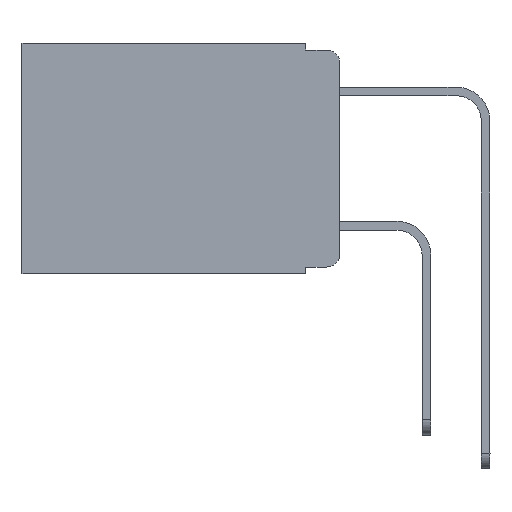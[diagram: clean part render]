
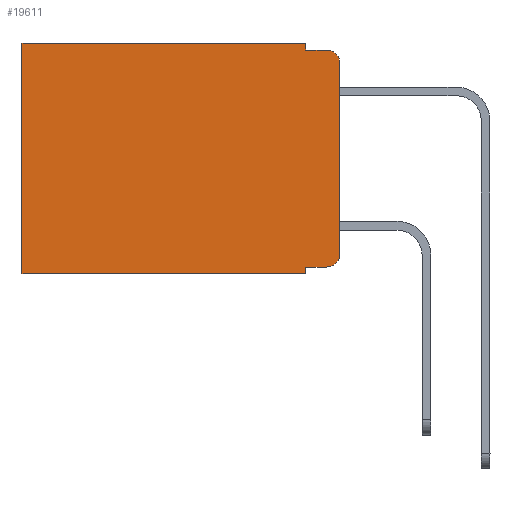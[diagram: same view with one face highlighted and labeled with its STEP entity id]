
A CAD part, left-side view. The second image highlights one B-rep face of the part: STEP entity #19611.
In plain terms, the highlighted planar face has unit normal (-1, 0, 0).
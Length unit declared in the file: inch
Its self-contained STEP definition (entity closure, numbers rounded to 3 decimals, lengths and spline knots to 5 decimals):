
#153 = VERTEX_POINT ( 'NONE', #23962 ) ;
#367 = ORIENTED_EDGE ( 'NONE', *, *, #16623, .T. ) ;
#507 = PLANE ( 'NONE',  #22811 ) ;
#697 = LINE ( 'NONE', #23389, #5428 ) ;
#757 = CARTESIAN_POINT ( 'NONE',  ( 0.298, 0., 0. ) ) ;
#948 = CIRCLE ( 'NONE', #19340, 0.02 ) ;
#1432 = CARTESIAN_POINT ( 'NONE',  ( 0.298, 0.051, -0.01 ) ) ;
#2094 = ORIENTED_EDGE ( 'NONE', *, *, #20021, .F. ) ;
#2096 = ORIENTED_EDGE ( 'NONE', *, *, #12876, .F. ) ;
#2594 = VECTOR ( 'NONE', #13783, 39.37008 ) ;
#2634 = DIRECTION ( 'NONE',  ( 0., 0., -1. ) ) ;
#2994 = DIRECTION ( 'NONE',  ( 0., 1., 0. ) ) ;
#3037 = ORIENTED_EDGE ( 'NONE', *, *, #12932, .F. ) ;
#3813 = CARTESIAN_POINT ( 'NONE',  ( 0.298, 0., -0.313 ) ) ;
#3879 = CARTESIAN_POINT ( 'NONE',  ( 0.298, 0.473, 0. ) ) ;
#4862 = ORIENTED_EDGE ( 'NONE', *, *, #23578, .T. ) ;
#5006 = DIRECTION ( 'NONE',  ( 0., 0., -1. ) ) ;
#5026 = VERTEX_POINT ( 'NONE', #20589 ) ;
#5389 = ORIENTED_EDGE ( 'NONE', *, *, #7988, .F. ) ;
#5428 = VECTOR ( 'NONE', #6217, 39.37008 ) ;
#6217 = DIRECTION ( 'NONE',  ( 0., 0., -1. ) ) ;
#7221 = VECTOR ( 'NONE', #14536, 39.37008 ) ;
#7294 = ORIENTED_EDGE ( 'NONE', *, *, #7670, .T. ) ;
#7316 = LINE ( 'NONE', #9185, #12214 ) ;
#7670 = EDGE_CURVE ( 'NONE', #18121, #22488, #16621, .T. ) ;
#7988 = EDGE_CURVE ( 'NONE', #23550, #10610, #697, .T. ) ;
#8569 = VECTOR ( 'NONE', #2994, 39.37008 ) ;
#8945 = CARTESIAN_POINT ( 'NONE',  ( 0.298, 0.02, -0.313 ) ) ;
#9013 = CARTESIAN_POINT ( 'NONE',  ( 0.298, 0.051, -0.333 ) ) ;
#9185 = CARTESIAN_POINT ( 'NONE',  ( 0.298, 0.051, 0. ) ) ;
#9774 = AXIS2_PLACEMENT_3D ( 'NONE', #8945, #14342, #22110 ) ;
#10610 = VERTEX_POINT ( 'NONE', #3813 ) ;
#10816 = CARTESIAN_POINT ( 'NONE',  ( 0.298, 0.051, -0.343 ) ) ;
#11115 = DIRECTION ( 'NONE',  ( -1., 0., 0. ) ) ;
#11215 = EDGE_CURVE ( 'NONE', #23550, #153, #948, .T. ) ;
#11369 = DIRECTION ( 'NONE',  ( 0., -1., 0. ) ) ;
#11825 = VERTEX_POINT ( 'NONE', #20735 ) ;
#12120 = EDGE_CURVE ( 'NONE', #5026, #10610, #13368, .T. ) ;
#12128 = CARTESIAN_POINT ( 'NONE',  ( 0.298, 0.473, 0. ) ) ;
#12143 = DIRECTION ( 'NONE',  ( 0., 0., -1. ) ) ;
#12171 = VERTEX_POINT ( 'NONE', #1432 ) ;
#12205 = VERTEX_POINT ( 'NONE', #10816 ) ;
#12214 = VECTOR ( 'NONE', #17088, 39.37008 ) ;
#12220 = EDGE_CURVE ( 'NONE', #12205, #13022, #24341, .T. ) ;
#12876 = EDGE_CURVE ( 'NONE', #18121, #12171, #7316, .T. ) ;
#12932 = EDGE_CURVE ( 'NONE', #11825, #12205, #22609, .T. ) ;
#13022 = VERTEX_POINT ( 'NONE', #19836 ) ;
#13068 = CARTESIAN_POINT ( 'NONE',  ( 0.298, 0.051, 0. ) ) ;
#13368 = CIRCLE ( 'NONE', #9774, 0.02 ) ;
#13783 = DIRECTION ( 'NONE',  ( 0., 1., 0. ) ) ;
#13907 = DIRECTION ( 'NONE',  ( 1., 0., 0. ) ) ;
#14342 = DIRECTION ( 'NONE',  ( -1., 0., 0. ) ) ;
#14536 = DIRECTION ( 'NONE',  ( 0., -1., 0. ) ) ;
#15395 = ORIENTED_EDGE ( 'NONE', *, *, #11215, .T. ) ;
#16378 = CARTESIAN_POINT ( 'NONE',  ( 0.298, 0., 0. ) ) ;
#16621 = LINE ( 'NONE', #16378, #8569 ) ;
#16623 = EDGE_CURVE ( 'NONE', #22488, #13022, #21647, .T. ) ;
#16649 = CARTESIAN_POINT ( 'NONE',  ( 0.298, 0.02, -0.03 ) ) ;
#16716 = CARTESIAN_POINT ( 'NONE',  ( 0.298, 0., -0.343 ) ) ;
#17088 = DIRECTION ( 'NONE',  ( 0., 0., -1. ) ) ;
#18121 = VERTEX_POINT ( 'NONE', #22320 ) ;
#18291 = VECTOR ( 'NONE', #2634, 39.37008 ) ;
#18297 = EDGE_LOOP ( 'NONE', ( #5389, #15395, #2094, #2096, #7294, #367, #23460, #3037, #4862, #19063 ) ) ;
#18652 = LINE ( 'NONE', #9013, #7221 ) ;
#18762 = CARTESIAN_POINT ( 'NONE',  ( 0.298, 0.051, -0.01 ) ) ;
#18773 = CARTESIAN_POINT ( 'NONE',  ( 0.298, 0., -0.03 ) ) ;
#19014 = LINE ( 'NONE', #18762, #23693 ) ;
#19063 = ORIENTED_EDGE ( 'NONE', *, *, #12120, .T. ) ;
#19340 = AXIS2_PLACEMENT_3D ( 'NONE', #16649, #11115, #5006 ) ;
#19611 = ADVANCED_FACE ( 'NONE', ( #21661 ), #507, .F. ) ;
#19836 = CARTESIAN_POINT ( 'NONE',  ( 0.298, 0.473, -0.343 ) ) ;
#20021 = EDGE_CURVE ( 'NONE', #12171, #153, #19014, .T. ) ;
#20589 = CARTESIAN_POINT ( 'NONE',  ( 0.298, 0.02, -0.333 ) ) ;
#20715 = DIRECTION ( 'NONE',  ( 0., 0., -1. ) ) ;
#20735 = CARTESIAN_POINT ( 'NONE',  ( 0.298, 0.051, -0.333 ) ) ;
#21414 = VECTOR ( 'NONE', #20715, 39.37008 ) ;
#21647 = LINE ( 'NONE', #12128, #18291 ) ;
#21661 = FACE_OUTER_BOUND ( 'NONE', #18297, .T. ) ;
#22110 = DIRECTION ( 'NONE',  ( 0., 0., -1. ) ) ;
#22320 = CARTESIAN_POINT ( 'NONE',  ( 0.298, 0.051, 0. ) ) ;
#22488 = VERTEX_POINT ( 'NONE', #3879 ) ;
#22609 = LINE ( 'NONE', #13068, #21414 ) ;
#22811 = AXIS2_PLACEMENT_3D ( 'NONE', #757, #13907, #12143 ) ;
#23389 = CARTESIAN_POINT ( 'NONE',  ( 0.298, 0., 0. ) ) ;
#23460 = ORIENTED_EDGE ( 'NONE', *, *, #12220, .F. ) ;
#23550 = VERTEX_POINT ( 'NONE', #18773 ) ;
#23578 = EDGE_CURVE ( 'NONE', #11825, #5026, #18652, .T. ) ;
#23693 = VECTOR ( 'NONE', #11369, 39.37008 ) ;
#23962 = CARTESIAN_POINT ( 'NONE',  ( 0.298, 0.02, -0.01 ) ) ;
#24341 = LINE ( 'NONE', #16716, #2594 ) ;
